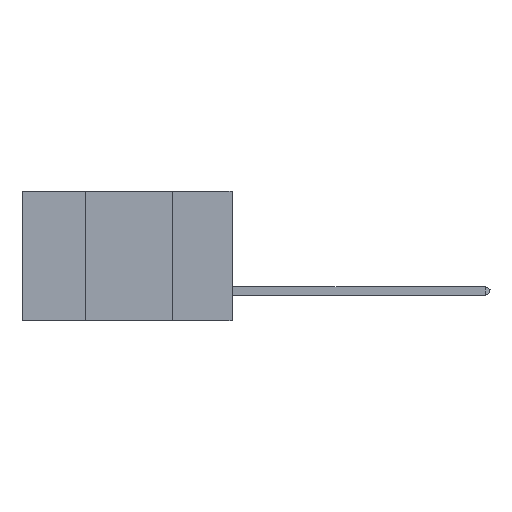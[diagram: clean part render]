
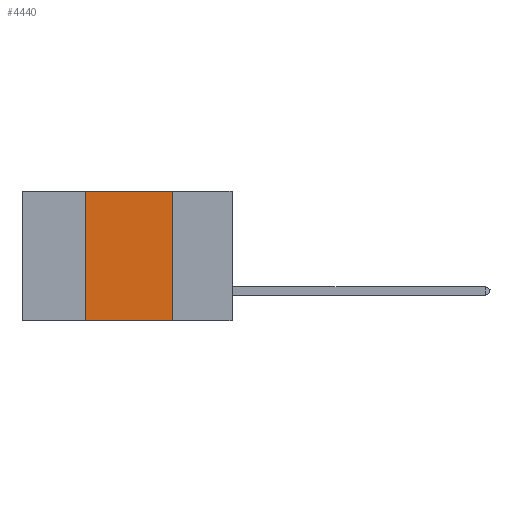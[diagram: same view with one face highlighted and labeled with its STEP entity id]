
A CAD part, left-side view. The second image highlights one B-rep face of the part: STEP entity #4440.
In plain terms, the highlighted planar face has unit normal (-1, 0, 0).
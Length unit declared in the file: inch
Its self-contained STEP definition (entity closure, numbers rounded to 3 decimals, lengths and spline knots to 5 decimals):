
#1518 = DIRECTION ( 'NONE',  ( 0., 0., 1. ) ) ;
#1640 = VECTOR ( 'NONE', #15398, 39.37008 ) ;
#1711 = CARTESIAN_POINT ( 'NONE',  ( 0., 0.42, 0. ) ) ;
#2436 = EDGE_CURVE ( 'NONE', #13414, #13126, #11207, .T. ) ;
#2578 = DIRECTION ( 'NONE',  ( 0., 0., -1. ) ) ;
#3880 = CARTESIAN_POINT ( 'NONE',  ( 0., 0.6, 0. ) ) ;
#4260 = PLANE ( 'NONE',  #9590 ) ;
#4440 = ADVANCED_FACE ( 'NONE', ( #8318 ), #4260, .F. ) ;
#5340 = VECTOR ( 'NONE', #15948, 39.37008 ) ;
#5544 = ORIENTED_EDGE ( 'NONE', *, *, #16472, .F. ) ;
#5869 = VECTOR ( 'NONE', #1518, 39.37008 ) ;
#6211 = LINE ( 'NONE', #3880, #1640 ) ;
#6358 = ORIENTED_EDGE ( 'NONE', *, *, #17680, .T. ) ;
#8169 = VERTEX_POINT ( 'NONE', #8410 ) ;
#8318 = FACE_OUTER_BOUND ( 'NONE', #13395, .T. ) ;
#8410 = CARTESIAN_POINT ( 'NONE',  ( 0., 0.17, -0.37 ) ) ;
#8679 = CARTESIAN_POINT ( 'NONE',  ( 0., 0.42, -0.37 ) ) ;
#9061 = CARTESIAN_POINT ( 'NONE',  ( 0., 0.17, 0. ) ) ;
#9590 = AXIS2_PLACEMENT_3D ( 'NONE', #11541, #11351, #2578 ) ;
#10072 = VECTOR ( 'NONE', #13549, 39.37008 ) ;
#11207 = LINE ( 'NONE', #1711, #5869 ) ;
#11351 = DIRECTION ( 'NONE',  ( 1., 0., 0. ) ) ;
#11541 = CARTESIAN_POINT ( 'NONE',  ( 0., 0.6, 0. ) ) ;
#12248 = CARTESIAN_POINT ( 'NONE',  ( 0., 0.6, -0.37 ) ) ;
#12952 = ORIENTED_EDGE ( 'NONE', *, *, #16083, .F. ) ;
#13126 = VERTEX_POINT ( 'NONE', #18875 ) ;
#13395 = EDGE_LOOP ( 'NONE', ( #12952, #5544, #13767, #6358 ) ) ;
#13414 = VERTEX_POINT ( 'NONE', #8679 ) ;
#13549 = DIRECTION ( 'NONE',  ( 0., -1., 0. ) ) ;
#13767 = ORIENTED_EDGE ( 'NONE', *, *, #2436, .F. ) ;
#15398 = DIRECTION ( 'NONE',  ( 0., -1., 0. ) ) ;
#15948 = DIRECTION ( 'NONE',  ( 0., 0., -1. ) ) ;
#16083 = EDGE_CURVE ( 'NONE', #17330, #8169, #18810, .T. ) ;
#16472 = EDGE_CURVE ( 'NONE', #13126, #17330, #6211, .T. ) ;
#17330 = VERTEX_POINT ( 'NONE', #9061 ) ;
#17680 = EDGE_CURVE ( 'NONE', #13414, #8169, #18952, .T. ) ;
#18810 = LINE ( 'NONE', #18900, #5340 ) ;
#18875 = CARTESIAN_POINT ( 'NONE',  ( 0., 0.42, 0. ) ) ;
#18900 = CARTESIAN_POINT ( 'NONE',  ( 0., 0.17, 0. ) ) ;
#18952 = LINE ( 'NONE', #12248, #10072 ) ;
